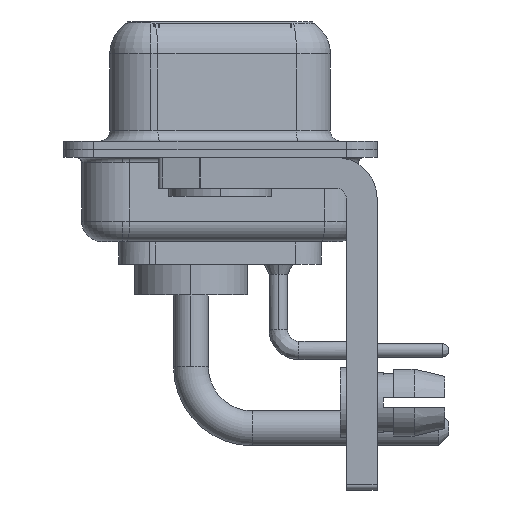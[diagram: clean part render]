
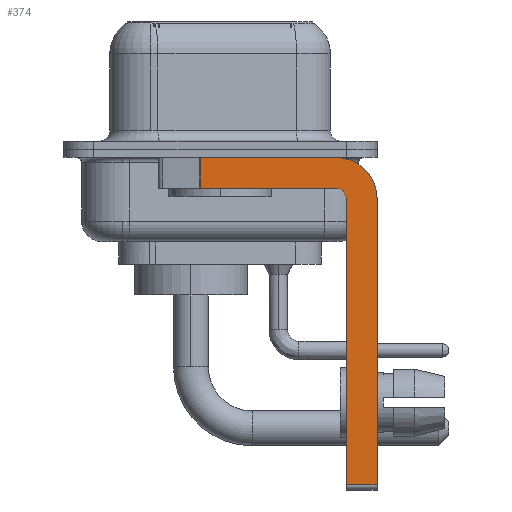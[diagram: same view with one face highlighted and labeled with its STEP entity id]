
A CAD part, left-side view. The second image highlights one B-rep face of the part: STEP entity #374.
In plain terms, the highlighted planar face has unit normal (-1, 0, 0).
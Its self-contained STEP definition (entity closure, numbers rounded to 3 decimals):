
#374 = ADVANCED_FACE ( 'NONE', ( #933 ), #14066, .F. ) ;
#422 = EDGE_CURVE ( 'NONE', #9487, #13854, #6888, .T. ) ;
#609 = ORIENTED_EDGE ( 'NONE', *, *, #20557, .F. ) ;
#933 = FACE_OUTER_BOUND ( 'NONE', #10522, .T. ) ;
#1220 = DIRECTION ( 'NONE',  ( 0., 0., 1. ) ) ;
#1680 = CIRCLE ( 'NONE', #22290, 0.5 ) ;
#2120 = VECTOR ( 'NONE', #23374, 1000. ) ;
#2295 = DIRECTION ( 'NONE',  ( 0., 0., 1. ) ) ;
#2705 = DIRECTION ( 'NONE',  ( 0., 0., -1. ) ) ;
#2742 = ORIENTED_EDGE ( 'NONE', *, *, #15113, .F. ) ;
#2943 = VERTEX_POINT ( 'NONE', #14762 ) ;
#3303 = CARTESIAN_POINT ( 'NONE',  ( -2.9, -6.15, -16.35 ) ) ;
#3314 = LINE ( 'NONE', #16098, #2120 ) ;
#3765 = VERTEX_POINT ( 'NONE', #7675 ) ;
#3875 = ORIENTED_EDGE ( 'NONE', *, *, #422, .T. ) ;
#4157 = EDGE_CURVE ( 'NONE', #9487, #22877, #5333, .T. ) ;
#4703 = EDGE_CURVE ( 'NONE', #23457, #3765, #20127, .T. ) ;
#5007 = EDGE_CURVE ( 'NONE', #13160, #2943, #1680, .T. ) ;
#5089 = CARTESIAN_POINT ( 'NONE',  ( -2.9, 0.978, -1.9 ) ) ;
#5317 = AXIS2_PLACEMENT_3D ( 'NONE', #21349, #15622, #23122 ) ;
#5333 = LINE ( 'NONE', #7130, #11214 ) ;
#6888 = LINE ( 'NONE', #5089, #15987 ) ;
#6982 = EDGE_CURVE ( 'NONE', #23457, #13160, #17234, .T. ) ;
#7130 = CARTESIAN_POINT ( 'NONE',  ( -2.9, 3., -0.4 ) ) ;
#7675 = CARTESIAN_POINT ( 'NONE',  ( -2.9, -7.65, -16.35 ) ) ;
#8146 = CARTESIAN_POINT ( 'NONE',  ( -2.9, -6.15, -16.6 ) ) ;
#8522 = CIRCLE ( 'NONE', #9683, 2. ) ;
#8633 = VERTEX_POINT ( 'NONE', #17938 ) ;
#8789 = CARTESIAN_POINT ( 'NONE',  ( -2.9, -6.15, -2.4 ) ) ;
#9487 = VERTEX_POINT ( 'NONE', #14150 ) ;
#9683 = AXIS2_PLACEMENT_3D ( 'NONE', #15834, #17623, #2705 ) ;
#10326 = DIRECTION ( 'NONE',  ( -1., 0., 0. ) ) ;
#10522 = EDGE_LOOP ( 'NONE', ( #18088, #3875, #609, #12927, #15127, #19310, #18429, #2742 ) ) ;
#10615 = VECTOR ( 'NONE', #21424, 1000. ) ;
#10974 = DIRECTION ( 'NONE',  ( 0., -1., 0. ) ) ;
#11214 = VECTOR ( 'NONE', #10974, 1000. ) ;
#12927 = ORIENTED_EDGE ( 'NONE', *, *, #5007, .F. ) ;
#13160 = VERTEX_POINT ( 'NONE', #8789 ) ;
#13854 = VERTEX_POINT ( 'NONE', #14596 ) ;
#14066 = PLANE ( 'NONE',  #5317 ) ;
#14149 = LINE ( 'NONE', #19630, #10615 ) ;
#14150 = CARTESIAN_POINT ( 'NONE',  ( -2.9, 0.978, -0.4 ) ) ;
#14596 = CARTESIAN_POINT ( 'NONE',  ( -2.9, 0.978, -1.9 ) ) ;
#14762 = CARTESIAN_POINT ( 'NONE',  ( -2.9, -5.65, -1.9 ) ) ;
#14982 = CARTESIAN_POINT ( 'NONE',  ( -2.9, -5.65, -16.35 ) ) ;
#15113 = EDGE_CURVE ( 'NONE', #22877, #8633, #8522, .T. ) ;
#15127 = ORIENTED_EDGE ( 'NONE', *, *, #6982, .F. ) ;
#15622 = DIRECTION ( 'NONE',  ( 1., 0., 0. ) ) ;
#15834 = CARTESIAN_POINT ( 'NONE',  ( -2.9, -5.65, -2.4 ) ) ;
#15987 = VECTOR ( 'NONE', #17637, 1000. ) ;
#16098 = CARTESIAN_POINT ( 'NONE',  ( -2.9, -7.65, -2.4 ) ) ;
#17234 = LINE ( 'NONE', #8146, #19316 ) ;
#17623 = DIRECTION ( 'NONE',  ( 1., 0., 0. ) ) ;
#17637 = DIRECTION ( 'NONE',  ( 0., 0., -1. ) ) ;
#17938 = CARTESIAN_POINT ( 'NONE',  ( -2.9, -7.65, -2.4 ) ) ;
#17952 = CARTESIAN_POINT ( 'NONE',  ( -2.9, -5.65, -2.4 ) ) ;
#18088 = ORIENTED_EDGE ( 'NONE', *, *, #4157, .F. ) ;
#18126 = EDGE_CURVE ( 'NONE', #8633, #3765, #3314, .T. ) ;
#18429 = ORIENTED_EDGE ( 'NONE', *, *, #18126, .F. ) ;
#18896 = CARTESIAN_POINT ( 'NONE',  ( -2.9, -5.65, -0.4 ) ) ;
#19310 = ORIENTED_EDGE ( 'NONE', *, *, #4703, .T. ) ;
#19316 = VECTOR ( 'NONE', #2295, 1000. ) ;
#19630 = CARTESIAN_POINT ( 'NONE',  ( -2.9, -5.65, -1.9 ) ) ;
#20127 = LINE ( 'NONE', #14982, #22273 ) ;
#20557 = EDGE_CURVE ( 'NONE', #2943, #13854, #14149, .T. ) ;
#21349 = CARTESIAN_POINT ( 'NONE',  ( -2.9, -5.65, -2.4 ) ) ;
#21424 = DIRECTION ( 'NONE',  ( 0., 1., 0. ) ) ;
#22264 = DIRECTION ( 'NONE',  ( 0., -1., 0. ) ) ;
#22273 = VECTOR ( 'NONE', #22264, 1000. ) ;
#22290 = AXIS2_PLACEMENT_3D ( 'NONE', #17952, #10326, #1220 ) ;
#22877 = VERTEX_POINT ( 'NONE', #18896 ) ;
#23122 = DIRECTION ( 'NONE',  ( 0., 0., -1. ) ) ;
#23374 = DIRECTION ( 'NONE',  ( 0., 0., -1. ) ) ;
#23457 = VERTEX_POINT ( 'NONE', #3303 ) ;
